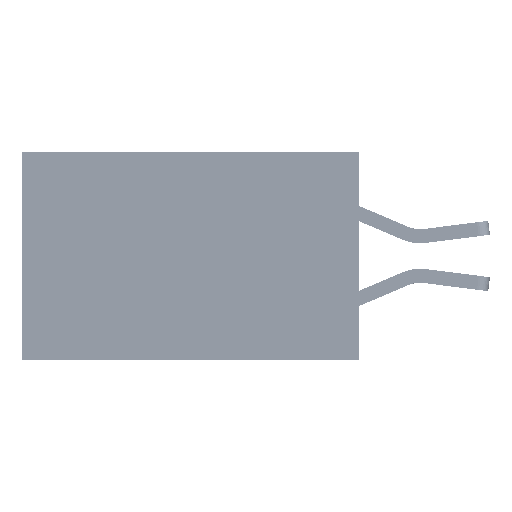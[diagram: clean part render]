
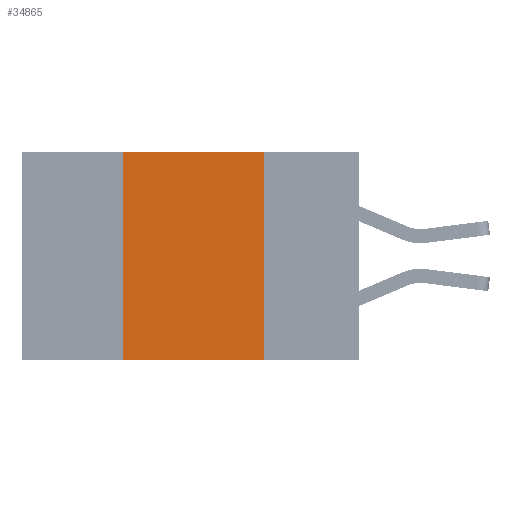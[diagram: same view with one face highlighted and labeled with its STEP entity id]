
A CAD part, left-side view. The second image highlights one B-rep face of the part: STEP entity #34865.
In plain terms, the highlighted planar face has unit normal (-1, 0, 0).
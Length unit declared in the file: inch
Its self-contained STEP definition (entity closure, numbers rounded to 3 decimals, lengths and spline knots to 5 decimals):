
#1615 = ORIENTED_EDGE ( 'NONE', *, *, #35904, .F. ) ;
#3238 = VERTEX_POINT ( 'NONE', #23020 ) ;
#5388 = PLANE ( 'NONE',  #22540 ) ;
#10495 = DIRECTION ( 'NONE',  ( 0., 0., 1. ) ) ;
#11004 = LINE ( 'NONE', #47495, #39617 ) ;
#11271 = VERTEX_POINT ( 'NONE', #13895 ) ;
#13895 = CARTESIAN_POINT ( 'NONE',  ( 0., 0.17, -0.37 ) ) ;
#14440 = CARTESIAN_POINT ( 'NONE',  ( 0., 0.6, 0. ) ) ;
#15914 = CARTESIAN_POINT ( 'NONE',  ( 0., 0.42, 0. ) ) ;
#17324 = DIRECTION ( 'NONE',  ( 1., 0., 0. ) ) ;
#18103 = VERTEX_POINT ( 'NONE', #15914 ) ;
#18437 = EDGE_CURVE ( 'NONE', #3238, #18103, #11004, .T. ) ;
#18667 = CARTESIAN_POINT ( 'NONE',  ( 0., 0.6, -0.37 ) ) ;
#20726 = EDGE_CURVE ( 'NONE', #25824, #11271, #27114, .T. ) ;
#21414 = CARTESIAN_POINT ( 'NONE',  ( 0., 0.17, 0. ) ) ;
#22540 = AXIS2_PLACEMENT_3D ( 'NONE', #31495, #17324, #39191 ) ;
#23020 = CARTESIAN_POINT ( 'NONE',  ( 0., 0.42, -0.37 ) ) ;
#23872 = DIRECTION ( 'NONE',  ( 0., 0., -1. ) ) ;
#24253 = EDGE_CURVE ( 'NONE', #3238, #11271, #40492, .T. ) ;
#25824 = VERTEX_POINT ( 'NONE', #21414 ) ;
#26813 = LINE ( 'NONE', #14440, #32014 ) ;
#27114 = LINE ( 'NONE', #34923, #46337 ) ;
#29422 = DIRECTION ( 'NONE',  ( 0., -1., 0. ) ) ;
#30155 = FACE_OUTER_BOUND ( 'NONE', #37714, .T. ) ;
#31495 = CARTESIAN_POINT ( 'NONE',  ( 0., 0.6, 0. ) ) ;
#32014 = VECTOR ( 'NONE', #48033, 39.37008 ) ;
#33990 = ORIENTED_EDGE ( 'NONE', *, *, #24253, .T. ) ;
#34267 = ORIENTED_EDGE ( 'NONE', *, *, #18437, .F. ) ;
#34865 = ADVANCED_FACE ( 'NONE', ( #30155 ), #5388, .F. ) ;
#34923 = CARTESIAN_POINT ( 'NONE',  ( 0., 0.17, 0. ) ) ;
#35904 = EDGE_CURVE ( 'NONE', #18103, #25824, #26813, .T. ) ;
#37714 = EDGE_LOOP ( 'NONE', ( #48267, #1615, #34267, #33990 ) ) ;
#39191 = DIRECTION ( 'NONE',  ( 0., 0., -1. ) ) ;
#39617 = VECTOR ( 'NONE', #10495, 39.37008 ) ;
#40492 = LINE ( 'NONE', #18667, #47460 ) ;
#46337 = VECTOR ( 'NONE', #23872, 39.37008 ) ;
#47460 = VECTOR ( 'NONE', #29422, 39.37008 ) ;
#47495 = CARTESIAN_POINT ( 'NONE',  ( 0., 0.42, 0. ) ) ;
#48033 = DIRECTION ( 'NONE',  ( 0., -1., 0. ) ) ;
#48267 = ORIENTED_EDGE ( 'NONE', *, *, #20726, .F. ) ;
